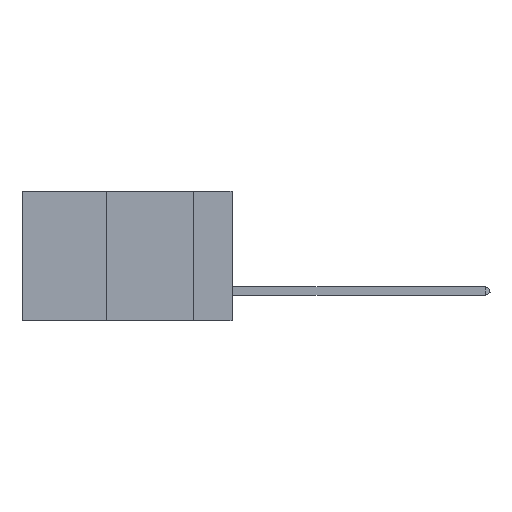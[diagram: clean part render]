
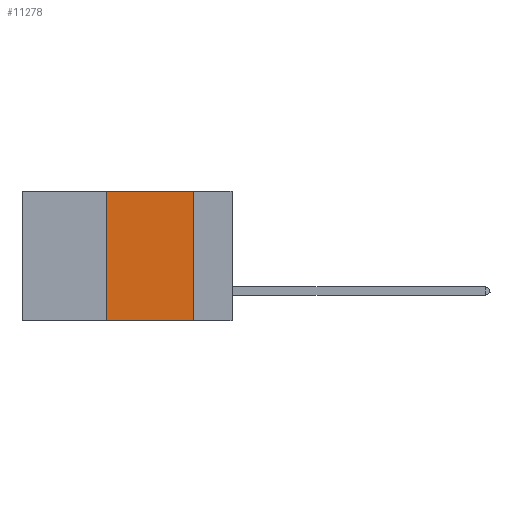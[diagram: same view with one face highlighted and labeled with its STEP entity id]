
A CAD part, left-side view. The second image highlights one B-rep face of the part: STEP entity #11278.
In plain terms, the highlighted planar face has unit normal (-1, 0, 0).
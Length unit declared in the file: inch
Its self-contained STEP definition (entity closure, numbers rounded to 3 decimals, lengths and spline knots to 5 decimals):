
#56 = DIRECTION ( 'NONE',  ( 0., -1., 0. ) ) ;
#1172 = AXIS2_PLACEMENT_3D ( 'NONE', #2835, #17886, #11776 ) ;
#1347 = DIRECTION ( 'NONE',  ( 0., -1., 0. ) ) ;
#2813 = LINE ( 'NONE', #17561, #5612 ) ;
#2835 = CARTESIAN_POINT ( 'NONE',  ( 0., 0.6, 0. ) ) ;
#3384 = VERTEX_POINT ( 'NONE', #17019 ) ;
#5079 = DIRECTION ( 'NONE',  ( 0., 0., 1. ) ) ;
#5367 = EDGE_CURVE ( 'NONE', #13433, #3384, #9420, .T. ) ;
#5612 = VECTOR ( 'NONE', #8654, 39.37008 ) ;
#5983 = ORIENTED_EDGE ( 'NONE', *, *, #7737, .F. ) ;
#6418 = LINE ( 'NONE', #15142, #17356 ) ;
#6479 = VERTEX_POINT ( 'NONE', #13641 ) ;
#6500 = ORIENTED_EDGE ( 'NONE', *, *, #16740, .F. ) ;
#7166 = EDGE_LOOP ( 'NONE', ( #5983, #6500, #16677, #17955 ) ) ;
#7620 = CARTESIAN_POINT ( 'NONE',  ( 0., 0.36, -0.37 ) ) ;
#7737 = EDGE_CURVE ( 'NONE', #8192, #6479, #2813, .T. ) ;
#7897 = LINE ( 'NONE', #19061, #18629 ) ;
#8192 = VERTEX_POINT ( 'NONE', #8234 ) ;
#8234 = CARTESIAN_POINT ( 'NONE',  ( 0., 0.11, 0. ) ) ;
#8654 = DIRECTION ( 'NONE',  ( 0., 0., -1. ) ) ;
#9420 = LINE ( 'NONE', #15772, #10586 ) ;
#10586 = VECTOR ( 'NONE', #5079, 39.37008 ) ;
#11278 = ADVANCED_FACE ( 'NONE', ( #13406 ), #12030, .F. ) ;
#11776 = DIRECTION ( 'NONE',  ( 0., 0., -1. ) ) ;
#12030 = PLANE ( 'NONE',  #1172 ) ;
#13406 = FACE_OUTER_BOUND ( 'NONE', #7166, .T. ) ;
#13433 = VERTEX_POINT ( 'NONE', #7620 ) ;
#13641 = CARTESIAN_POINT ( 'NONE',  ( 0., 0.11, -0.37 ) ) ;
#15142 = CARTESIAN_POINT ( 'NONE',  ( 0., 0.6, -0.37 ) ) ;
#15772 = CARTESIAN_POINT ( 'NONE',  ( 0., 0.36, 0. ) ) ;
#16677 = ORIENTED_EDGE ( 'NONE', *, *, #5367, .F. ) ;
#16740 = EDGE_CURVE ( 'NONE', #3384, #8192, #7897, .T. ) ;
#17019 = CARTESIAN_POINT ( 'NONE',  ( 0., 0.36, 0. ) ) ;
#17356 = VECTOR ( 'NONE', #56, 39.37008 ) ;
#17561 = CARTESIAN_POINT ( 'NONE',  ( 0., 0.11, 0. ) ) ;
#17886 = DIRECTION ( 'NONE',  ( 1., 0., 0. ) ) ;
#17955 = ORIENTED_EDGE ( 'NONE', *, *, #18484, .T. ) ;
#18484 = EDGE_CURVE ( 'NONE', #13433, #6479, #6418, .T. ) ;
#18629 = VECTOR ( 'NONE', #1347, 39.37008 ) ;
#19061 = CARTESIAN_POINT ( 'NONE',  ( 0., 0.6, 0. ) ) ;
